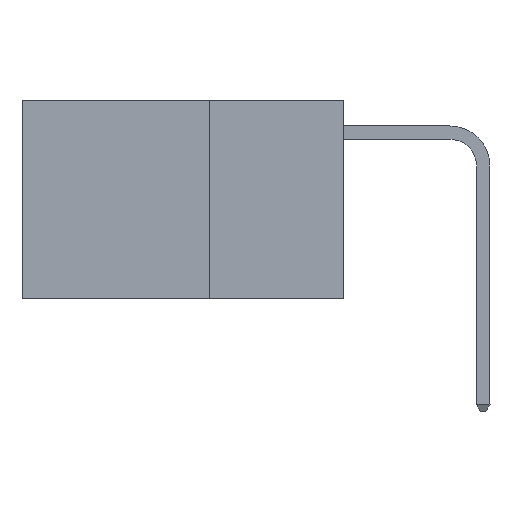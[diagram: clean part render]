
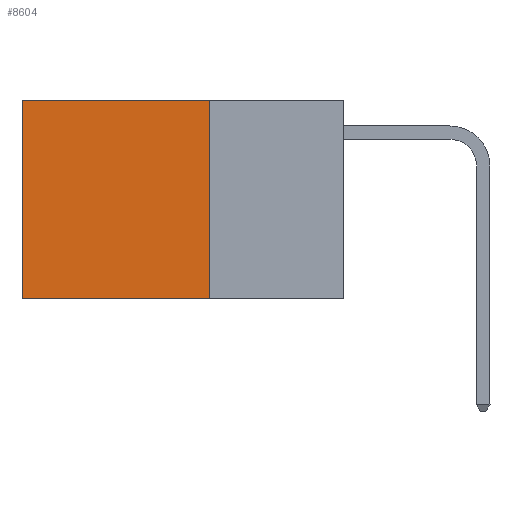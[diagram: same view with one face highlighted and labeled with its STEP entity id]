
A CAD part, left-side view. The second image highlights one B-rep face of the part: STEP entity #8604.
In plain terms, the highlighted planar face has unit normal (-1, 0, 0).
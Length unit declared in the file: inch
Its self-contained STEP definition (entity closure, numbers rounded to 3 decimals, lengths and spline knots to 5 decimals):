
#316 = VERTEX_POINT ( 'NONE', #3122 ) ;
#439 = DIRECTION ( 'NONE',  ( 0., 0., -1. ) ) ;
#1353 = DIRECTION ( 'NONE',  ( 0., 0., -1. ) ) ;
#1424 = CARTESIAN_POINT ( 'NONE',  ( 0.2625, 0.25, 0. ) ) ;
#1515 = CARTESIAN_POINT ( 'NONE',  ( 0.2625, 0.6, 0. ) ) ;
#1628 = CARTESIAN_POINT ( 'NONE',  ( 0.2625, 0.25, -0.37 ) ) ;
#1660 = EDGE_LOOP ( 'NONE', ( #11780, #2029, #2548, #5063 ) ) ;
#2029 = ORIENTED_EDGE ( 'NONE', *, *, #13155, .F. ) ;
#2162 = DIRECTION ( 'NONE',  ( 0., 0., -1. ) ) ;
#2548 = ORIENTED_EDGE ( 'NONE', *, *, #13806, .F. ) ;
#2564 = CARTESIAN_POINT ( 'NONE',  ( 0.2625, 0.25, -0.37 ) ) ;
#3122 = CARTESIAN_POINT ( 'NONE',  ( 0.2625, 0.25, 0. ) ) ;
#3302 = CARTESIAN_POINT ( 'NONE',  ( 0.2625, 0.6, -0.37 ) ) ;
#3401 = CARTESIAN_POINT ( 'NONE',  ( 0.2625, 0.25, 0. ) ) ;
#3687 = VECTOR ( 'NONE', #15914, 39.37008 ) ;
#4331 = VERTEX_POINT ( 'NONE', #1515 ) ;
#5063 = ORIENTED_EDGE ( 'NONE', *, *, #12589, .T. ) ;
#6019 = DIRECTION ( 'NONE',  ( 1., 0., 0. ) ) ;
#6048 = VECTOR ( 'NONE', #7997, 39.37008 ) ;
#6185 = LINE ( 'NONE', #16079, #3687 ) ;
#7896 = CARTESIAN_POINT ( 'NONE',  ( 0.2625, 0.6, 0. ) ) ;
#7997 = DIRECTION ( 'NONE',  ( 0., 1., 0. ) ) ;
#8604 = ADVANCED_FACE ( 'NONE', ( #10671 ), #14601, .F. ) ;
#9886 = EDGE_CURVE ( 'NONE', #4331, #11756, #15507, .T. ) ;
#10354 = AXIS2_PLACEMENT_3D ( 'NONE', #3401, #6019, #2162 ) ;
#10671 = FACE_OUTER_BOUND ( 'NONE', #1660, .T. ) ;
#11563 = VERTEX_POINT ( 'NONE', #2564 ) ;
#11756 = VERTEX_POINT ( 'NONE', #3302 ) ;
#11780 = ORIENTED_EDGE ( 'NONE', *, *, #9886, .T. ) ;
#12278 = VECTOR ( 'NONE', #1353, 39.37008 ) ;
#12589 = EDGE_CURVE ( 'NONE', #316, #4331, #6185, .T. ) ;
#13155 = EDGE_CURVE ( 'NONE', #11563, #11756, #14149, .T. ) ;
#13786 = VECTOR ( 'NONE', #439, 39.37008 ) ;
#13806 = EDGE_CURVE ( 'NONE', #316, #11563, #14025, .T. ) ;
#14025 = LINE ( 'NONE', #1424, #12278 ) ;
#14149 = LINE ( 'NONE', #1628, #6048 ) ;
#14601 = PLANE ( 'NONE',  #10354 ) ;
#15507 = LINE ( 'NONE', #7896, #13786 ) ;
#15914 = DIRECTION ( 'NONE',  ( 0., 1., 0. ) ) ;
#16079 = CARTESIAN_POINT ( 'NONE',  ( 0.2625, 0.25, 0. ) ) ;
